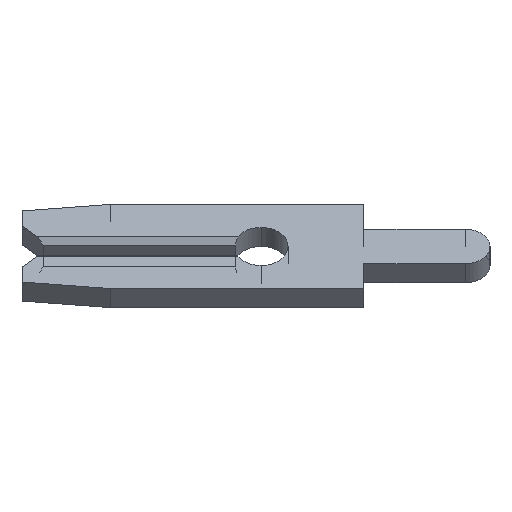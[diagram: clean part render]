
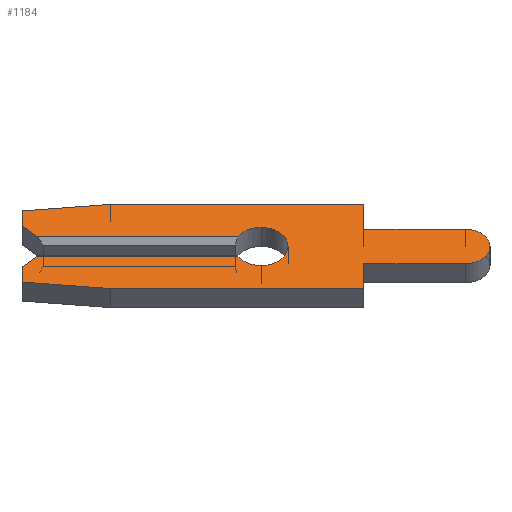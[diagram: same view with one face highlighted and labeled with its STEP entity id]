
A CAD part, left-side view. The second image highlights one B-rep face of the part: STEP entity #1184.
In plain terms, the highlighted face is planar.
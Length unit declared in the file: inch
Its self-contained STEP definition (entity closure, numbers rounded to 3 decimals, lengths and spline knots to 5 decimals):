
#2 = VERTEX_POINT ( 'NONE', #1961 ) ;
#13 = ORIENTED_EDGE ( 'NONE', *, *, #551, .T. ) ;
#15 = AXIS2_PLACEMENT_3D ( 'NONE', #1296, #394, #575 ) ;
#34 = DIRECTION ( 'NONE',  ( 0., -0.707, 0.707 ) ) ;
#38 = CARTESIAN_POINT ( 'NONE',  ( -0.013, 0., -0.026 ) ) ;
#43 = EDGE_CURVE ( 'NONE', #1041, #1909, #2139, .T. ) ;
#81 = CARTESIAN_POINT ( 'NONE',  ( -0.013, 0.231, 0.04857 ) ) ;
#88 = CARTESIAN_POINT ( 'NONE',  ( -0.013, 0.231, 0.028 ) ) ;
#97 = CARTESIAN_POINT ( 'NONE',  ( -0.013, 0.216, 0.013 ) ) ;
#121 = CARTESIAN_POINT ( 'NONE',  ( -0.013, -0.099, -0.0235 ) ) ;
#124 = ORIENTED_EDGE ( 'NONE', *, *, #362, .F. ) ;
#130 = LINE ( 'NONE', #81, #935 ) ;
#142 = CARTESIAN_POINT ( 'NONE',  ( -0.013, 0.216, -0.013 ) ) ;
#240 = LINE ( 'NONE', #1390, #2025 ) ;
#241 = EDGE_CURVE ( 'NONE', #2112, #2169, #2077, .T. ) ;
#245 = CIRCLE ( 'NONE', #410, 0.026 ) ;
#252 = DIRECTION ( 'NONE',  ( -1., 0., 0. ) ) ;
#288 = DIRECTION ( 'NONE',  ( 0., -0.995, 0.105 ) ) ;
#294 = DIRECTION ( 'NONE',  ( 0., 1., 0. ) ) ;
#322 = EDGE_CURVE ( 'NONE', #1504, #441, #2218, .T. ) ;
#340 = AXIS2_PLACEMENT_3D ( 'NONE', #818, #252, #435 ) ;
#362 = EDGE_CURVE ( 'NONE', #1819, #2346, #1840, .T. ) ;
#381 = LINE ( 'NONE', #552, #2114 ) ;
#394 = DIRECTION ( 'NONE',  ( 1., 0., 0. ) ) ;
#410 = AXIS2_PLACEMENT_3D ( 'NONE', #2027, #1484, #1279 ) ;
#435 = DIRECTION ( 'NONE',  ( 0., 0., -1. ) ) ;
#441 = VERTEX_POINT ( 'NONE', #2042 ) ;
#446 = CIRCLE ( 'NONE', #1789, 0.026 ) ;
#551 = EDGE_CURVE ( 'NONE', #1415, #2, #700, .T. ) ;
#552 = CARTESIAN_POINT ( 'NONE',  ( -0.013, 0.146, -0.0575 ) ) ;
#558 = CARTESIAN_POINT ( 'NONE',  ( -0.013, 0.02252, -0.013 ) ) ;
#575 = DIRECTION ( 'NONE',  ( 0., 0., 1. ) ) ;
#595 = EDGE_CURVE ( 'NONE', #2346, #1041, #245, .T. ) ;
#614 = ORIENTED_EDGE ( 'NONE', *, *, #1153, .F. ) ;
#616 = LINE ( 'NONE', #2291, #2313 ) ;
#628 = DIRECTION ( 'NONE',  ( 0., 0.707, 0.707 ) ) ;
#640 = CARTESIAN_POINT ( 'NONE',  ( -0.013, -0.1975, 0.0235 ) ) ;
#672 = EDGE_CURVE ( 'NONE', #1413, #1103, #2091, .T. ) ;
#675 = LINE ( 'NONE', #2244, #1137 ) ;
#696 = EDGE_LOOP ( 'NONE', ( #13, #925, #1589, #1195, #124, #1529, #1585, #1474, #1645, #1797, #1324, #1847, #926, #614, #2224, #1254, #1992, #1068 ) ) ;
#700 = LINE ( 'NONE', #901, #2118 ) ;
#762 = VECTOR ( 'NONE', #628, 39.37008 ) ;
#817 = LINE ( 'NONE', #1163, #1013 ) ;
#818 = CARTESIAN_POINT ( 'NONE',  ( -0.013, 0., 0. ) ) ;
#842 = VERTEX_POINT ( 'NONE', #1716 ) ;
#860 = CARTESIAN_POINT ( 'NONE',  ( -0.013, -0.099, 0.0235 ) ) ;
#894 = CARTESIAN_POINT ( 'NONE',  ( -0.013, -0.099, -0.0575 ) ) ;
#896 = EDGE_CURVE ( 'NONE', #441, #1819, #675, .T. ) ;
#900 = CARTESIAN_POINT ( 'NONE',  ( -0.013, -0.099, 0.0575 ) ) ;
#901 = CARTESIAN_POINT ( 'NONE',  ( -0.013, 0.231, 0.013 ) ) ;
#925 = ORIENTED_EDGE ( 'NONE', *, *, #1232, .F. ) ;
#926 = ORIENTED_EDGE ( 'NONE', *, *, #1275, .F. ) ;
#935 = VECTOR ( 'NONE', #288, 39.37008 ) ;
#982 = DIRECTION ( 'NONE',  ( 0., -1., 0. ) ) ;
#999 = CARTESIAN_POINT ( 'NONE',  ( -0.013, 0., 0. ) ) ;
#1012 = DIRECTION ( 'NONE',  ( 0., 0., -1. ) ) ;
#1013 = VECTOR ( 'NONE', #1167, 39.37008 ) ;
#1023 = CARTESIAN_POINT ( 'NONE',  ( -0.013, 0.231, -0.04857 ) ) ;
#1041 = VERTEX_POINT ( 'NONE', #38 ) ;
#1068 = ORIENTED_EDGE ( 'NONE', *, *, #1173, .F. ) ;
#1096 = VECTOR ( 'NONE', #1274, 39.37008 ) ;
#1103 = VERTEX_POINT ( 'NONE', #1894 ) ;
#1137 = VECTOR ( 'NONE', #34, 39.37008 ) ;
#1153 = EDGE_CURVE ( 'NONE', #2169, #1501, #817, .T. ) ;
#1160 = AXIS2_PLACEMENT_3D ( 'NONE', #999, #1913, #1012 ) ;
#1163 = CARTESIAN_POINT ( 'NONE',  ( -0.013, -0.099, 0.0575 ) ) ;
#1167 = DIRECTION ( 'NONE',  ( 0., 0., -1. ) ) ;
#1173 = EDGE_CURVE ( 'NONE', #1415, #2255, #1440, .T. ) ;
#1184 = ADVANCED_FACE ( 'NONE', ( #1911 ), #1756, .F. ) ;
#1195 = ORIENTED_EDGE ( 'NONE', *, *, #595, .F. ) ;
#1228 = LINE ( 'NONE', #1934, #1823 ) ;
#1232 = EDGE_CURVE ( 'NONE', #1909, #2, #446, .T. ) ;
#1254 = ORIENTED_EDGE ( 'NONE', *, *, #1290, .F. ) ;
#1274 = DIRECTION ( 'NONE',  ( 0., -1., 0. ) ) ;
#1275 = EDGE_CURVE ( 'NONE', #1501, #1413, #616, .T. ) ;
#1278 = DIRECTION ( 'NONE',  ( 0., 1., 0. ) ) ;
#1279 = DIRECTION ( 'NONE',  ( 0., 0., -1. ) ) ;
#1290 = EDGE_CURVE ( 'NONE', #842, #2112, #130, .T. ) ;
#1296 = CARTESIAN_POINT ( 'NONE',  ( -0.013, -0.1975, 0. ) ) ;
#1324 = ORIENTED_EDGE ( 'NONE', *, *, #1563, .F. ) ;
#1332 = EDGE_CURVE ( 'NONE', #1614, #1504, #1228, .T. ) ;
#1372 = DIRECTION ( 'NONE',  ( 0., 0., 1. ) ) ;
#1384 = DIRECTION ( 'NONE',  ( 0., 0.995, 0.105 ) ) ;
#1390 = CARTESIAN_POINT ( 'NONE',  ( -0.013, -0.099, -0.0235 ) ) ;
#1413 = VERTEX_POINT ( 'NONE', #640 ) ;
#1415 = VERTEX_POINT ( 'NONE', #97 ) ;
#1426 = DIRECTION ( 'NONE',  ( 0., -1., 0. ) ) ;
#1440 = LINE ( 'NONE', #2274, #762 ) ;
#1454 = EDGE_CURVE ( 'NONE', #2255, #842, #1477, .T. ) ;
#1456 = CARTESIAN_POINT ( 'NONE',  ( -0.013, 0.146, 0.0575 ) ) ;
#1474 = ORIENTED_EDGE ( 'NONE', *, *, #1332, .F. ) ;
#1477 = LINE ( 'NONE', #88, #2087 ) ;
#1484 = DIRECTION ( 'NONE',  ( -1., 0., 0. ) ) ;
#1501 = VERTEX_POINT ( 'NONE', #860 ) ;
#1504 = VERTEX_POINT ( 'NONE', #1023 ) ;
#1529 = ORIENTED_EDGE ( 'NONE', *, *, #896, .F. ) ;
#1563 = EDGE_CURVE ( 'NONE', #1103, #1591, #240, .T. ) ;
#1585 = ORIENTED_EDGE ( 'NONE', *, *, #322, .F. ) ;
#1589 = ORIENTED_EDGE ( 'NONE', *, *, #43, .F. ) ;
#1591 = VERTEX_POINT ( 'NONE', #121 ) ;
#1614 = VERTEX_POINT ( 'NONE', #1772 ) ;
#1630 = CARTESIAN_POINT ( 'NONE',  ( -0.013, 0., 0.026 ) ) ;
#1641 = CARTESIAN_POINT ( 'NONE',  ( -0.013, 0.231, -0.028 ) ) ;
#1645 = ORIENTED_EDGE ( 'NONE', *, *, #1885, .F. ) ;
#1652 = CARTESIAN_POINT ( 'NONE',  ( -0.013, -0.099, -0.0575 ) ) ;
#1668 = DIRECTION ( 'NONE',  ( 0., -1., 0. ) ) ;
#1677 = LINE ( 'NONE', #894, #1902 ) ;
#1716 = CARTESIAN_POINT ( 'NONE',  ( -0.013, 0.231, 0.04857 ) ) ;
#1733 = VECTOR ( 'NONE', #1977, 39.37008 ) ;
#1756 = PLANE ( 'NONE',  #1160 ) ;
#1764 = DIRECTION ( 'NONE',  ( 0., 0., -1. ) ) ;
#1772 = CARTESIAN_POINT ( 'NONE',  ( -0.013, 0.146, -0.0575 ) ) ;
#1789 = AXIS2_PLACEMENT_3D ( 'NONE', #2107, #2129, #1764 ) ;
#1797 = ORIENTED_EDGE ( 'NONE', *, *, #1966, .F. ) ;
#1819 = VERTEX_POINT ( 'NONE', #142 ) ;
#1823 = VECTOR ( 'NONE', #1384, 39.37008 ) ;
#1840 = LINE ( 'NONE', #2012, #2162 ) ;
#1847 = ORIENTED_EDGE ( 'NONE', *, *, #672, .F. ) ;
#1885 = EDGE_CURVE ( 'NONE', #1962, #1614, #381, .T. ) ;
#1894 = CARTESIAN_POINT ( 'NONE',  ( -0.013, -0.1975, -0.0235 ) ) ;
#1902 = VECTOR ( 'NONE', #1981, 39.37008 ) ;
#1909 = VERTEX_POINT ( 'NONE', #1630 ) ;
#1911 = FACE_OUTER_BOUND ( 'NONE', #696, .T. ) ;
#1913 = DIRECTION ( 'NONE',  ( 1., 0., 0. ) ) ;
#1934 = CARTESIAN_POINT ( 'NONE',  ( -0.013, 0.231, -0.04857 ) ) ;
#1961 = CARTESIAN_POINT ( 'NONE',  ( -0.013, 0.02252, 0.013 ) ) ;
#1962 = VERTEX_POINT ( 'NONE', #1652 ) ;
#1966 = EDGE_CURVE ( 'NONE', #1591, #1962, #1677, .T. ) ;
#1977 = DIRECTION ( 'NONE',  ( 0., 0., 1. ) ) ;
#1981 = DIRECTION ( 'NONE',  ( 0., 0., -1. ) ) ;
#1992 = ORIENTED_EDGE ( 'NONE', *, *, #1454, .F. ) ;
#2012 = CARTESIAN_POINT ( 'NONE',  ( -0.013, 0., -0.013 ) ) ;
#2025 = VECTOR ( 'NONE', #294, 39.37008 ) ;
#2027 = CARTESIAN_POINT ( 'NONE',  ( -0.013, 0., 0. ) ) ;
#2042 = CARTESIAN_POINT ( 'NONE',  ( -0.013, 0.231, -0.028 ) ) ;
#2077 = LINE ( 'NONE', #2180, #1096 ) ;
#2087 = VECTOR ( 'NONE', #1372, 39.37008 ) ;
#2091 = CIRCLE ( 'NONE', #15, 0.0235 ) ;
#2107 = CARTESIAN_POINT ( 'NONE',  ( -0.013, 0., 0. ) ) ;
#2112 = VERTEX_POINT ( 'NONE', #1456 ) ;
#2114 = VECTOR ( 'NONE', #1278, 39.37008 ) ;
#2118 = VECTOR ( 'NONE', #1668, 39.37008 ) ;
#2129 = DIRECTION ( 'NONE',  ( -1., 0., 0. ) ) ;
#2139 = CIRCLE ( 'NONE', #340, 0.026 ) ;
#2162 = VECTOR ( 'NONE', #1426, 39.37008 ) ;
#2169 = VERTEX_POINT ( 'NONE', #900 ) ;
#2180 = CARTESIAN_POINT ( 'NONE',  ( -0.013, 0.146, 0.0575 ) ) ;
#2203 = CARTESIAN_POINT ( 'NONE',  ( -0.013, 0.231, 0.028 ) ) ;
#2218 = LINE ( 'NONE', #1641, #1733 ) ;
#2224 = ORIENTED_EDGE ( 'NONE', *, *, #241, .F. ) ;
#2244 = CARTESIAN_POINT ( 'NONE',  ( -0.013, 0.2105, -0.0075 ) ) ;
#2255 = VERTEX_POINT ( 'NONE', #2203 ) ;
#2274 = CARTESIAN_POINT ( 'NONE',  ( -0.013, 0.2105, 0.0075 ) ) ;
#2291 = CARTESIAN_POINT ( 'NONE',  ( -0.013, -0.099, 0.0235 ) ) ;
#2313 = VECTOR ( 'NONE', #982, 39.37008 ) ;
#2346 = VERTEX_POINT ( 'NONE', #558 ) ;
